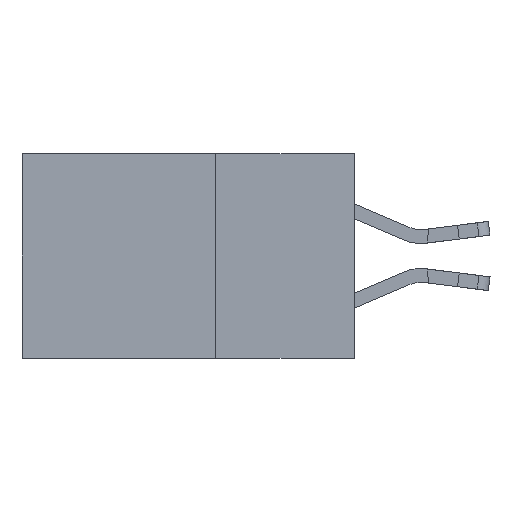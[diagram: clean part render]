
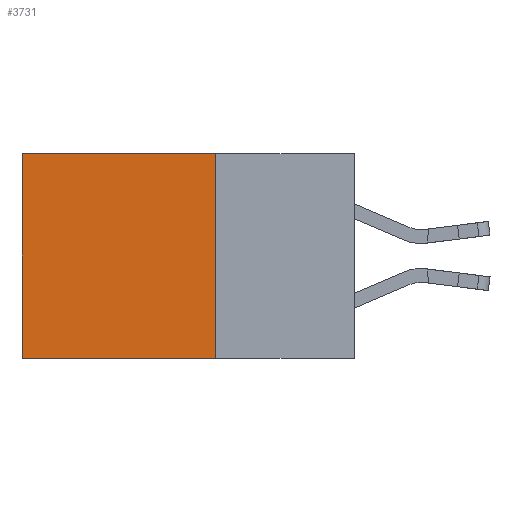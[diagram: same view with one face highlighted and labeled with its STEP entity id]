
A CAD part, left-side view. The second image highlights one B-rep face of the part: STEP entity #3731.
In plain terms, the highlighted planar face has unit normal (-1, 0, 0).
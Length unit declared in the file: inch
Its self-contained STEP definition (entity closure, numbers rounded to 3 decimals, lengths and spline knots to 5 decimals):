
#539 = PLANE ( 'NONE',  #18148 ) ;
#1017 = VERTEX_POINT ( 'NONE', #18188 ) ;
#1206 = VECTOR ( 'NONE', #16211, 39.37008 ) ;
#1243 = CARTESIAN_POINT ( 'NONE',  ( 0.298, 0.25, 0. ) ) ;
#3456 = ORIENTED_EDGE ( 'NONE', *, *, #5126, .T. ) ;
#3731 = ADVANCED_FACE ( 'NONE', ( #5786 ), #539, .F. ) ;
#4332 = VERTEX_POINT ( 'NONE', #17724 ) ;
#5126 = EDGE_CURVE ( 'NONE', #20543, #12199, #6343, .T. ) ;
#5736 = ORIENTED_EDGE ( 'NONE', *, *, #13149, .F. ) ;
#5786 = FACE_OUTER_BOUND ( 'NONE', #25393, .T. ) ;
#6274 = CARTESIAN_POINT ( 'NONE',  ( 0.298, 0.25, -0.37 ) ) ;
#6343 = LINE ( 'NONE', #1243, #20958 ) ;
#6380 = LINE ( 'NONE', #24008, #10157 ) ;
#7425 = DIRECTION ( 'NONE',  ( 0., 1., 0. ) ) ;
#9029 = EDGE_CURVE ( 'NONE', #12199, #4332, #6380, .T. ) ;
#9143 = CARTESIAN_POINT ( 'NONE',  ( 0.298, 0.6, 0. ) ) ;
#9563 = ORIENTED_EDGE ( 'NONE', *, *, #18508, .F. ) ;
#9760 = ORIENTED_EDGE ( 'NONE', *, *, #9029, .T. ) ;
#10052 = CARTESIAN_POINT ( 'NONE',  ( 0.298, 0.25, 0. ) ) ;
#10157 = VECTOR ( 'NONE', #14076, 39.37008 ) ;
#10211 = VECTOR ( 'NONE', #10636, 39.37008 ) ;
#10636 = DIRECTION ( 'NONE',  ( 0., 1., 0. ) ) ;
#12199 = VERTEX_POINT ( 'NONE', #9143 ) ;
#12621 = DIRECTION ( 'NONE',  ( 1., 0., 0. ) ) ;
#13149 = EDGE_CURVE ( 'NONE', #20543, #1017, #19537, .T. ) ;
#14076 = DIRECTION ( 'NONE',  ( 0., 0., -1. ) ) ;
#14386 = CARTESIAN_POINT ( 'NONE',  ( 0.298, 0.25, 0. ) ) ;
#14641 = DIRECTION ( 'NONE',  ( 0., 0., -1. ) ) ;
#16211 = DIRECTION ( 'NONE',  ( 0., 0., -1. ) ) ;
#16730 = CARTESIAN_POINT ( 'NONE',  ( 0.298, 0.25, 0. ) ) ;
#17724 = CARTESIAN_POINT ( 'NONE',  ( 0.298, 0.6, -0.37 ) ) ;
#18148 = AXIS2_PLACEMENT_3D ( 'NONE', #16730, #12621, #14641 ) ;
#18188 = CARTESIAN_POINT ( 'NONE',  ( 0.298, 0.25, -0.37 ) ) ;
#18508 = EDGE_CURVE ( 'NONE', #1017, #4332, #22600, .T. ) ;
#19537 = LINE ( 'NONE', #14386, #1206 ) ;
#20543 = VERTEX_POINT ( 'NONE', #10052 ) ;
#20958 = VECTOR ( 'NONE', #7425, 39.37008 ) ;
#22600 = LINE ( 'NONE', #6274, #10211 ) ;
#24008 = CARTESIAN_POINT ( 'NONE',  ( 0.298, 0.6, 0. ) ) ;
#25393 = EDGE_LOOP ( 'NONE', ( #9760, #9563, #5736, #3456 ) ) ;
